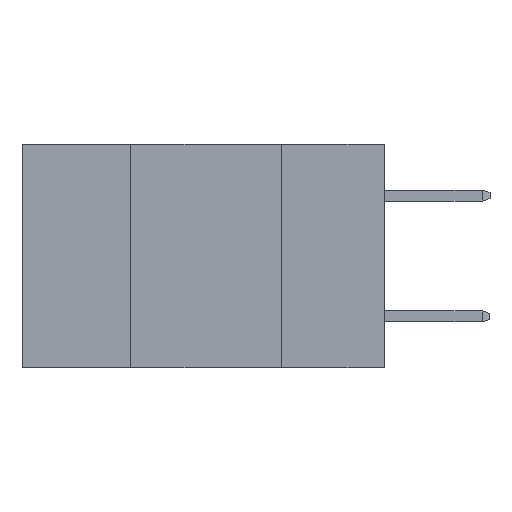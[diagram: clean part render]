
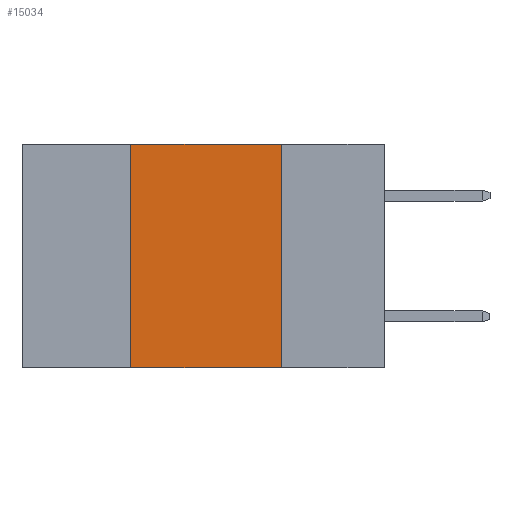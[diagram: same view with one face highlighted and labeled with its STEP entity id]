
A CAD part, left-side view. The second image highlights one B-rep face of the part: STEP entity #15034.
In plain terms, the highlighted planar face has unit normal (-1, 0, 0).
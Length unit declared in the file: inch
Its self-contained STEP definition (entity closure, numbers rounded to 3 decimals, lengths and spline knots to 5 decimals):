
#860 = VECTOR ( 'NONE', #17108, 39.37008 ) ;
#895 = ORIENTED_EDGE ( 'NONE', *, *, #1540, .F. ) ;
#1424 = VECTOR ( 'NONE', #14775, 39.37008 ) ;
#1540 = EDGE_CURVE ( 'NONE', #2882, #14011, #15205, .T. ) ;
#1941 = ORIENTED_EDGE ( 'NONE', *, *, #3437, .F. ) ;
#2312 = VERTEX_POINT ( 'NONE', #19743 ) ;
#2882 = VERTEX_POINT ( 'NONE', #8081 ) ;
#3437 = EDGE_CURVE ( 'NONE', #2312, #2882, #13227, .T. ) ;
#3537 = ORIENTED_EDGE ( 'NONE', *, *, #9357, .F. ) ;
#3953 = VECTOR ( 'NONE', #4409, 39.37008 ) ;
#4409 = DIRECTION ( 'NONE',  ( 0., 0., 1. ) ) ;
#5425 = PLANE ( 'NONE',  #6349 ) ;
#6256 = LINE ( 'NONE', #13280, #1424 ) ;
#6349 = AXIS2_PLACEMENT_3D ( 'NONE', #15889, #6923, #17384 ) ;
#6923 = DIRECTION ( 'NONE',  ( 1., 0., 0. ) ) ;
#8081 = CARTESIAN_POINT ( 'NONE',  ( 0., 0.17, 0. ) ) ;
#8507 = FACE_OUTER_BOUND ( 'NONE', #18610, .T. ) ;
#8775 = ORIENTED_EDGE ( 'NONE', *, *, #12787, .T. ) ;
#9357 = EDGE_CURVE ( 'NONE', #17863, #2312, #11561, .T. ) ;
#9519 = CARTESIAN_POINT ( 'NONE',  ( 0., 0.17, -0.37 ) ) ;
#11255 = VECTOR ( 'NONE', #11280, 39.37008 ) ;
#11280 = DIRECTION ( 'NONE',  ( 0., 0., -1. ) ) ;
#11561 = LINE ( 'NONE', #13421, #3953 ) ;
#12787 = EDGE_CURVE ( 'NONE', #17863, #14011, #6256, .T. ) ;
#13227 = LINE ( 'NONE', #16296, #860 ) ;
#13280 = CARTESIAN_POINT ( 'NONE',  ( 0., 0.6, -0.37 ) ) ;
#13421 = CARTESIAN_POINT ( 'NONE',  ( 0., 0.42, 0. ) ) ;
#14011 = VERTEX_POINT ( 'NONE', #9519 ) ;
#14775 = DIRECTION ( 'NONE',  ( 0., -1., 0. ) ) ;
#15034 = ADVANCED_FACE ( 'NONE', ( #8507 ), #5425, .F. ) ;
#15205 = LINE ( 'NONE', #15843, #11255 ) ;
#15843 = CARTESIAN_POINT ( 'NONE',  ( 0., 0.17, 0. ) ) ;
#15889 = CARTESIAN_POINT ( 'NONE',  ( 0., 0.6, 0. ) ) ;
#15995 = CARTESIAN_POINT ( 'NONE',  ( 0., 0.42, -0.37 ) ) ;
#16296 = CARTESIAN_POINT ( 'NONE',  ( 0., 0.6, 0. ) ) ;
#17108 = DIRECTION ( 'NONE',  ( 0., -1., 0. ) ) ;
#17384 = DIRECTION ( 'NONE',  ( 0., 0., -1. ) ) ;
#17863 = VERTEX_POINT ( 'NONE', #15995 ) ;
#18610 = EDGE_LOOP ( 'NONE', ( #895, #1941, #3537, #8775 ) ) ;
#19743 = CARTESIAN_POINT ( 'NONE',  ( 0., 0.42, 0. ) ) ;
